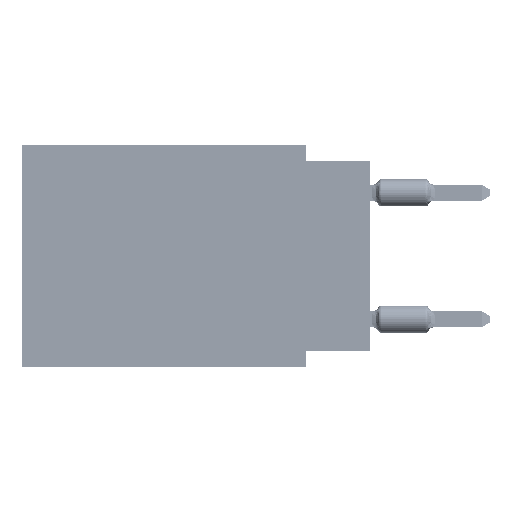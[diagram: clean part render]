
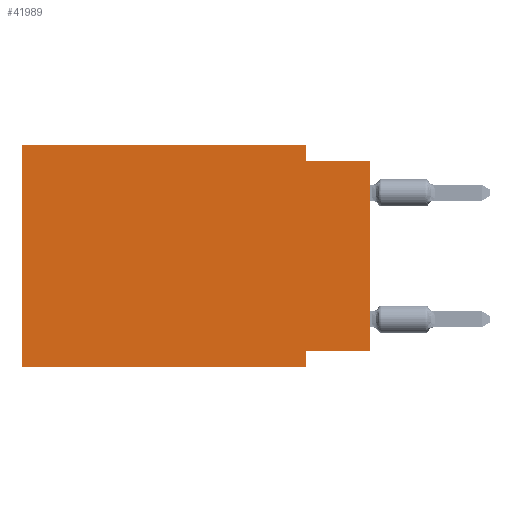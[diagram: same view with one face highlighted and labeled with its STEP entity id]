
A CAD part, left-side view. The second image highlights one B-rep face of the part: STEP entity #41989.
In plain terms, the highlighted planar face has unit normal (-1, 0, 0).
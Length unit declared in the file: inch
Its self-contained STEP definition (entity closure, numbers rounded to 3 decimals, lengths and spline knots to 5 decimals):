
#885 = CARTESIAN_POINT ( 'NONE',  ( 0., 0.1, -0.35 ) ) ;
#1304 = DIRECTION ( 'NONE',  ( 0., -1., 0. ) ) ;
#3051 = CARTESIAN_POINT ( 'NONE',  ( 0., 0., -0.325 ) ) ;
#3454 = EDGE_LOOP ( 'NONE', ( #7518, #45723, #19573, #75802, #14865, #55591, #43356, #56445 ) ) ;
#7124 = DIRECTION ( 'NONE',  ( 0., -1., 0. ) ) ;
#7423 = LINE ( 'NONE', #18718, #49508 ) ;
#7518 = ORIENTED_EDGE ( 'NONE', *, *, #49720, .T. ) ;
#8627 = VERTEX_POINT ( 'NONE', #53624 ) ;
#9143 = VERTEX_POINT ( 'NONE', #26586 ) ;
#11422 = VECTOR ( 'NONE', #7124, 39.37008 ) ;
#12563 = CARTESIAN_POINT ( 'NONE',  ( 0., 0., -0.025 ) ) ;
#14865 = ORIENTED_EDGE ( 'NONE', *, *, #63225, .F. ) ;
#14984 = VECTOR ( 'NONE', #49110, 39.37008 ) ;
#16053 = CARTESIAN_POINT ( 'NONE',  ( 0., 0.1, -0.35 ) ) ;
#18718 = CARTESIAN_POINT ( 'NONE',  ( 0., 0., -0.325 ) ) ;
#19108 = DIRECTION ( 'NONE',  ( 0., 1., 0. ) ) ;
#19573 = ORIENTED_EDGE ( 'NONE', *, *, #27559, .F. ) ;
#19700 = VERTEX_POINT ( 'NONE', #74850 ) ;
#22335 = DIRECTION ( 'NONE',  ( 1., 0., 0. ) ) ;
#22514 = VERTEX_POINT ( 'NONE', #3051 ) ;
#22576 = DIRECTION ( 'NONE',  ( 0., 0., 1. ) ) ;
#23958 = EDGE_CURVE ( 'NONE', #19700, #44701, #58881, .T. ) ;
#24673 = CARTESIAN_POINT ( 'NONE',  ( 0., 0.55, -0.35 ) ) ;
#25018 = CARTESIAN_POINT ( 'NONE',  ( 0., 0.55, 0. ) ) ;
#25566 = VERTEX_POINT ( 'NONE', #16053 ) ;
#26539 = CARTESIAN_POINT ( 'NONE',  ( 0., 0.1, 0. ) ) ;
#26586 = CARTESIAN_POINT ( 'NONE',  ( 0., 0.1, -0.325 ) ) ;
#26911 = LINE ( 'NONE', #26539, #34696 ) ;
#27397 = PLANE ( 'NONE',  #54498 ) ;
#27559 = EDGE_CURVE ( 'NONE', #44701, #65843, #26911, .T. ) ;
#34696 = VECTOR ( 'NONE', #73224, 39.37008 ) ;
#34986 = LINE ( 'NONE', #47052, #42884 ) ;
#38191 = CARTESIAN_POINT ( 'NONE',  ( 0., 0.55, -0.35 ) ) ;
#39304 = EDGE_CURVE ( 'NONE', #9143, #25566, #54154, .T. ) ;
#41989 = ADVANCED_FACE ( 'NONE', ( #70181 ), #27397, .F. ) ;
#42087 = DIRECTION ( 'NONE',  ( 0., 0., -1. ) ) ;
#42160 = EDGE_CURVE ( 'NONE', #22514, #9143, #7423, .T. ) ;
#42884 = VECTOR ( 'NONE', #22576, 39.37008 ) ;
#43356 = ORIENTED_EDGE ( 'NONE', *, *, #39304, .F. ) ;
#44701 = VERTEX_POINT ( 'NONE', #51762 ) ;
#45723 = ORIENTED_EDGE ( 'NONE', *, *, #74075, .F. ) ;
#45771 = EDGE_CURVE ( 'NONE', #72447, #25566, #67769, .T. ) ;
#47052 = CARTESIAN_POINT ( 'NONE',  ( 0., 0.55, 0. ) ) ;
#49110 = DIRECTION ( 'NONE',  ( 0., -1., 0. ) ) ;
#49508 = VECTOR ( 'NONE', #19108, 39.37008 ) ;
#49720 = EDGE_CURVE ( 'NONE', #22514, #8627, #61985, .T. ) ;
#50682 = DIRECTION ( 'NONE',  ( 0., 0., 1. ) ) ;
#51762 = CARTESIAN_POINT ( 'NONE',  ( 0., 0.1, 0. ) ) ;
#53624 = CARTESIAN_POINT ( 'NONE',  ( 0., 0., -0.025 ) ) ;
#54154 = LINE ( 'NONE', #885, #56883 ) ;
#54498 = AXIS2_PLACEMENT_3D ( 'NONE', #68626, #22335, #69021 ) ;
#55591 = ORIENTED_EDGE ( 'NONE', *, *, #45771, .T. ) ;
#56445 = ORIENTED_EDGE ( 'NONE', *, *, #42160, .F. ) ;
#56883 = VECTOR ( 'NONE', #42087, 39.37008 ) ;
#58881 = LINE ( 'NONE', #25018, #73142 ) ;
#61985 = LINE ( 'NONE', #62759, #62529 ) ;
#62529 = VECTOR ( 'NONE', #50682, 39.37008 ) ;
#62759 = CARTESIAN_POINT ( 'NONE',  ( 0., 0., 0. ) ) ;
#63225 = EDGE_CURVE ( 'NONE', #72447, #19700, #34986, .T. ) ;
#65843 = VERTEX_POINT ( 'NONE', #70817 ) ;
#67769 = LINE ( 'NONE', #38191, #14984 ) ;
#68626 = CARTESIAN_POINT ( 'NONE',  ( 0., 0.55, 0. ) ) ;
#69021 = DIRECTION ( 'NONE',  ( 0., 0., -1. ) ) ;
#70181 = FACE_OUTER_BOUND ( 'NONE', #3454, .T. ) ;
#70817 = CARTESIAN_POINT ( 'NONE',  ( 0., 0.1, -0.025 ) ) ;
#72447 = VERTEX_POINT ( 'NONE', #24673 ) ;
#73142 = VECTOR ( 'NONE', #1304, 39.37008 ) ;
#73209 = LINE ( 'NONE', #12563, #11422 ) ;
#73224 = DIRECTION ( 'NONE',  ( 0., 0., -1. ) ) ;
#74075 = EDGE_CURVE ( 'NONE', #65843, #8627, #73209, .T. ) ;
#74850 = CARTESIAN_POINT ( 'NONE',  ( 0., 0.55, 0. ) ) ;
#75802 = ORIENTED_EDGE ( 'NONE', *, *, #23958, .F. ) ;
